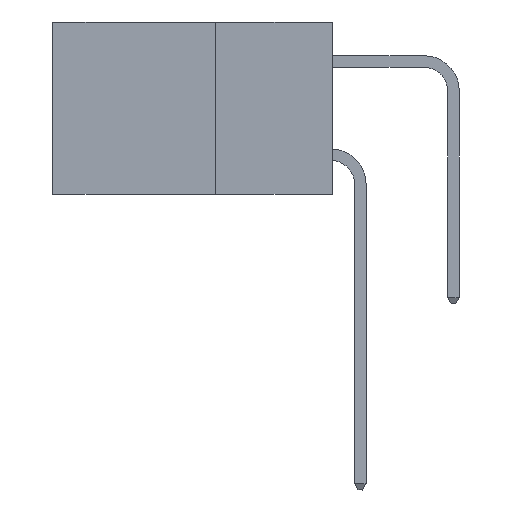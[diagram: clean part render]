
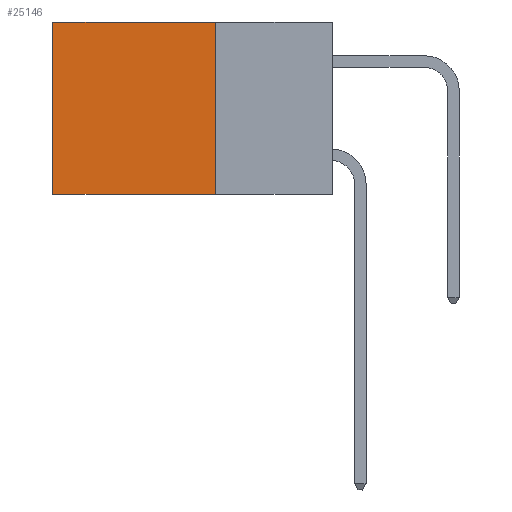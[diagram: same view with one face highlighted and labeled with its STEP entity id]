
A CAD part, left-side view. The second image highlights one B-rep face of the part: STEP entity #25146.
In plain terms, the highlighted planar face has unit normal (-1, 0, 0).
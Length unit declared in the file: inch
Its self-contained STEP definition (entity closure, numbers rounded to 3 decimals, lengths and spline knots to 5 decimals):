
#370 = VERTEX_POINT ( 'NONE', #10926 ) ;
#1783 = CARTESIAN_POINT ( 'NONE',  ( 0.298, 0.6, 0. ) ) ;
#2804 = CARTESIAN_POINT ( 'NONE',  ( 0.298, 0.25, -0.37 ) ) ;
#2990 = DIRECTION ( 'NONE',  ( 0., 0., -1. ) ) ;
#4236 = VERTEX_POINT ( 'NONE', #1783 ) ;
#5523 = EDGE_CURVE ( 'NONE', #370, #4236, #8965, .T. ) ;
#6100 = DIRECTION ( 'NONE',  ( 1., 0., 0. ) ) ;
#6715 = ORIENTED_EDGE ( 'NONE', *, *, #14913, .T. ) ;
#6848 = EDGE_CURVE ( 'NONE', #20896, #21496, #22147, .T. ) ;
#7085 = FACE_OUTER_BOUND ( 'NONE', #12943, .T. ) ;
#7722 = VECTOR ( 'NONE', #2990, 39.37008 ) ;
#8036 = ORIENTED_EDGE ( 'NONE', *, *, #5523, .T. ) ;
#8224 = VECTOR ( 'NONE', #21842, 39.37008 ) ;
#8965 = LINE ( 'NONE', #22410, #8224 ) ;
#9225 = LINE ( 'NONE', #14785, #21054 ) ;
#10926 = CARTESIAN_POINT ( 'NONE',  ( 0.298, 0.25, 0. ) ) ;
#12943 = EDGE_LOOP ( 'NONE', ( #6715, #24784, #20204, #8036 ) ) ;
#13126 = CARTESIAN_POINT ( 'NONE',  ( 0.298, 0.25, 0. ) ) ;
#13711 = EDGE_CURVE ( 'NONE', #370, #20896, #9225, .T. ) ;
#14398 = VECTOR ( 'NONE', #24123, 39.37008 ) ;
#14785 = CARTESIAN_POINT ( 'NONE',  ( 0.298, 0.25, 0. ) ) ;
#14844 = CARTESIAN_POINT ( 'NONE',  ( 0.298, 0.6, 0. ) ) ;
#14913 = EDGE_CURVE ( 'NONE', #4236, #21496, #21032, .T. ) ;
#17184 = DIRECTION ( 'NONE',  ( 0., 0., -1. ) ) ;
#20204 = ORIENTED_EDGE ( 'NONE', *, *, #13711, .F. ) ;
#20283 = PLANE ( 'NONE',  #20392 ) ;
#20392 = AXIS2_PLACEMENT_3D ( 'NONE', #13126, #6100, #22628 ) ;
#20896 = VERTEX_POINT ( 'NONE', #27389 ) ;
#21032 = LINE ( 'NONE', #14844, #7722 ) ;
#21054 = VECTOR ( 'NONE', #17184, 39.37008 ) ;
#21496 = VERTEX_POINT ( 'NONE', #24636 ) ;
#21842 = DIRECTION ( 'NONE',  ( 0., 1., 0. ) ) ;
#22147 = LINE ( 'NONE', #2804, #14398 ) ;
#22410 = CARTESIAN_POINT ( 'NONE',  ( 0.298, 0.25, 0. ) ) ;
#22628 = DIRECTION ( 'NONE',  ( 0., 0., -1. ) ) ;
#24123 = DIRECTION ( 'NONE',  ( 0., 1., 0. ) ) ;
#24636 = CARTESIAN_POINT ( 'NONE',  ( 0.298, 0.6, -0.37 ) ) ;
#24784 = ORIENTED_EDGE ( 'NONE', *, *, #6848, .F. ) ;
#25146 = ADVANCED_FACE ( 'NONE', ( #7085 ), #20283, .F. ) ;
#27389 = CARTESIAN_POINT ( 'NONE',  ( 0.298, 0.25, -0.37 ) ) ;
